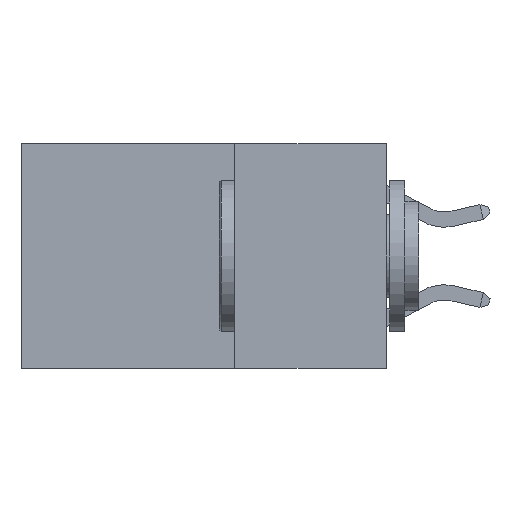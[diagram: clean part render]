
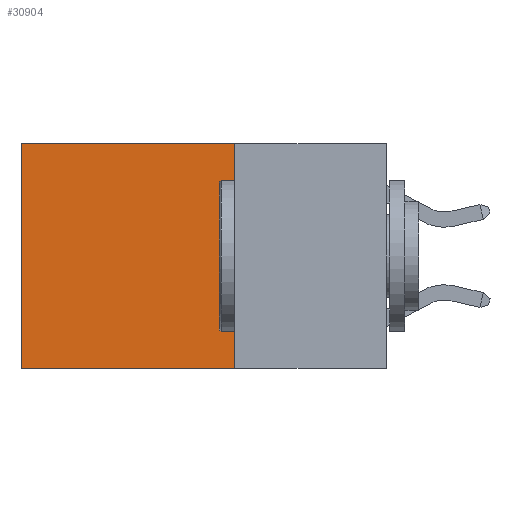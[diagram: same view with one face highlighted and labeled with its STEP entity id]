
A CAD part, left-side view. The second image highlights one B-rep face of the part: STEP entity #30904.
In plain terms, the highlighted planar face has unit normal (-1, 0, 0).
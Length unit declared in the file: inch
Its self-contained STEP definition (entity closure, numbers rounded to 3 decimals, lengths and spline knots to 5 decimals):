
#624 = DIRECTION ( 'NONE',  ( 0., 1., 0. ) ) ;
#2568 = EDGE_CURVE ( 'NONE', #6495, #25644, #10850, .T. ) ;
#2727 = CARTESIAN_POINT ( 'NONE',  ( 0.2625, 0.25, 0. ) ) ;
#3585 = CARTESIAN_POINT ( 'NONE',  ( 0.2625, 0.25, 0. ) ) ;
#4134 = EDGE_CURVE ( 'NONE', #6495, #20994, #5868, .T. ) ;
#5104 = CARTESIAN_POINT ( 'NONE',  ( 0.2625, 0.6, 0. ) ) ;
#5860 = DIRECTION ( 'NONE',  ( 0., 1., 0. ) ) ;
#5868 = LINE ( 'NONE', #2727, #27270 ) ;
#5980 = CARTESIAN_POINT ( 'NONE',  ( 0.2625, 0.25, 0. ) ) ;
#6495 = VERTEX_POINT ( 'NONE', #5980 ) ;
#9050 = PLANE ( 'NONE',  #26234 ) ;
#9282 = DIRECTION ( 'NONE',  ( 0., 0., -1. ) ) ;
#10850 = LINE ( 'NONE', #15668, #23935 ) ;
#11044 = ORIENTED_EDGE ( 'NONE', *, *, #4134, .F. ) ;
#13494 = CARTESIAN_POINT ( 'NONE',  ( 0.2625, 0.25, -0.37 ) ) ;
#14181 = ORIENTED_EDGE ( 'NONE', *, *, #2568, .T. ) ;
#15668 = CARTESIAN_POINT ( 'NONE',  ( 0.2625, 0.25, 0. ) ) ;
#16025 = EDGE_CURVE ( 'NONE', #20994, #21169, #21101, .T. ) ;
#16967 = CARTESIAN_POINT ( 'NONE',  ( 0.2625, 0.6, -0.37 ) ) ;
#18188 = DIRECTION ( 'NONE',  ( 0., 0., -1. ) ) ;
#19451 = VECTOR ( 'NONE', #9282, 39.37008 ) ;
#20994 = VERTEX_POINT ( 'NONE', #13494 ) ;
#21101 = LINE ( 'NONE', #26285, #27397 ) ;
#21169 = VERTEX_POINT ( 'NONE', #16967 ) ;
#21952 = LINE ( 'NONE', #32118, #19451 ) ;
#23935 = VECTOR ( 'NONE', #5860, 39.37008 ) ;
#25644 = VERTEX_POINT ( 'NONE', #5104 ) ;
#26234 = AXIS2_PLACEMENT_3D ( 'NONE', #3585, #29377, #26243 ) ;
#26243 = DIRECTION ( 'NONE',  ( 0., 0., -1. ) ) ;
#26285 = CARTESIAN_POINT ( 'NONE',  ( 0.2625, 0.25, -0.37 ) ) ;
#27270 = VECTOR ( 'NONE', #18188, 39.37008 ) ;
#27397 = VECTOR ( 'NONE', #624, 39.37008 ) ;
#28302 = EDGE_LOOP ( 'NONE', ( #30609, #29686, #11044, #14181 ) ) ;
#28618 = EDGE_CURVE ( 'NONE', #25644, #21169, #21952, .T. ) ;
#29377 = DIRECTION ( 'NONE',  ( 1., 0., 0. ) ) ;
#29686 = ORIENTED_EDGE ( 'NONE', *, *, #16025, .F. ) ;
#30609 = ORIENTED_EDGE ( 'NONE', *, *, #28618, .T. ) ;
#30904 = ADVANCED_FACE ( 'NONE', ( #31898 ), #9050, .F. ) ;
#31898 = FACE_OUTER_BOUND ( 'NONE', #28302, .T. ) ;
#32118 = CARTESIAN_POINT ( 'NONE',  ( 0.2625, 0.6, 0. ) ) ;
